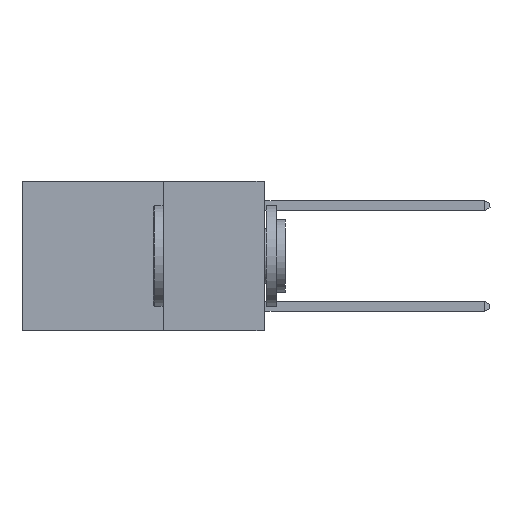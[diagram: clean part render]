
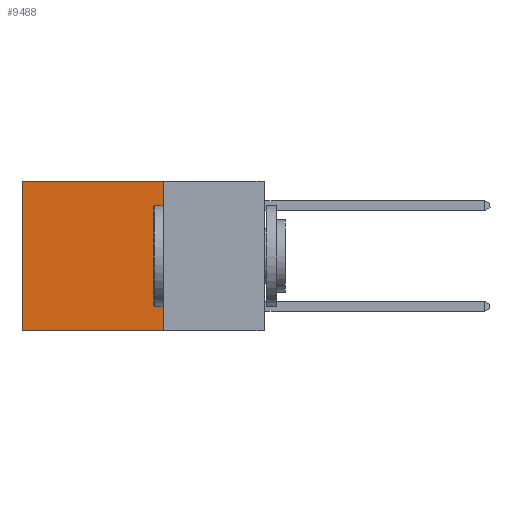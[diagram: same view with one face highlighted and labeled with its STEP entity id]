
A CAD part, left-side view. The second image highlights one B-rep face of the part: STEP entity #9488.
In plain terms, the highlighted planar face has unit normal (-1, 0, 0).
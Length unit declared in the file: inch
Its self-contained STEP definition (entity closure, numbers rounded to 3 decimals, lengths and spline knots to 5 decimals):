
#1 = EDGE_LOOP ( 'NONE', ( #2013, #5647, #11503, #2041 ) ) ;
#136 = PLANE ( 'NONE',  #7016 ) ;
#433 = CARTESIAN_POINT ( 'NONE',  ( 0.2625, 0.25, -0.37 ) ) ;
#486 = LINE ( 'NONE', #1902, #9659 ) ;
#656 = CARTESIAN_POINT ( 'NONE',  ( 0.2625, 0.25, 0. ) ) ;
#1111 = DIRECTION ( 'NONE',  ( 1., 0., 0. ) ) ;
#1433 = VERTEX_POINT ( 'NONE', #10335 ) ;
#1570 = DIRECTION ( 'NONE',  ( 0., 0., -1. ) ) ;
#1646 = CARTESIAN_POINT ( 'NONE',  ( 0.2625, 0.6, 0. ) ) ;
#1902 = CARTESIAN_POINT ( 'NONE',  ( 0.2625, 0.25, 0. ) ) ;
#1989 = DIRECTION ( 'NONE',  ( 0., 0., -1. ) ) ;
#2013 = ORIENTED_EDGE ( 'NONE', *, *, #2565, .T. ) ;
#2041 = ORIENTED_EDGE ( 'NONE', *, *, #6273, .T. ) ;
#2051 = CARTESIAN_POINT ( 'NONE',  ( 0.2625, 0.6, 0. ) ) ;
#2287 = VECTOR ( 'NONE', #8540, 39.37008 ) ;
#2565 = EDGE_CURVE ( 'NONE', #5335, #7854, #7817, .T. ) ;
#2802 = LINE ( 'NONE', #656, #4933 ) ;
#3999 = EDGE_CURVE ( 'NONE', #1433, #7854, #4845, .T. ) ;
#4308 = CARTESIAN_POINT ( 'NONE',  ( 0.2625, 0.25, 0. ) ) ;
#4845 = LINE ( 'NONE', #433, #2287 ) ;
#4933 = VECTOR ( 'NONE', #4989, 39.37008 ) ;
#4989 = DIRECTION ( 'NONE',  ( 0., 1., 0. ) ) ;
#5335 = VERTEX_POINT ( 'NONE', #2051 ) ;
#5647 = ORIENTED_EDGE ( 'NONE', *, *, #3999, .F. ) ;
#6273 = EDGE_CURVE ( 'NONE', #9767, #5335, #2802, .T. ) ;
#7016 = AXIS2_PLACEMENT_3D ( 'NONE', #9127, #1111, #1989 ) ;
#7817 = LINE ( 'NONE', #1646, #9170 ) ;
#7854 = VERTEX_POINT ( 'NONE', #10286 ) ;
#8540 = DIRECTION ( 'NONE',  ( 0., 1., 0. ) ) ;
#9113 = DIRECTION ( 'NONE',  ( 0., 0., -1. ) ) ;
#9127 = CARTESIAN_POINT ( 'NONE',  ( 0.2625, 0.25, 0. ) ) ;
#9170 = VECTOR ( 'NONE', #1570, 39.37008 ) ;
#9488 = ADVANCED_FACE ( 'NONE', ( #10008 ), #136, .F. ) ;
#9659 = VECTOR ( 'NONE', #9113, 39.37008 ) ;
#9767 = VERTEX_POINT ( 'NONE', #4308 ) ;
#10008 = FACE_OUTER_BOUND ( 'NONE', #1, .T. ) ;
#10233 = EDGE_CURVE ( 'NONE', #9767, #1433, #486, .T. ) ;
#10286 = CARTESIAN_POINT ( 'NONE',  ( 0.2625, 0.6, -0.37 ) ) ;
#10335 = CARTESIAN_POINT ( 'NONE',  ( 0.2625, 0.25, -0.37 ) ) ;
#11503 = ORIENTED_EDGE ( 'NONE', *, *, #10233, .F. ) ;
